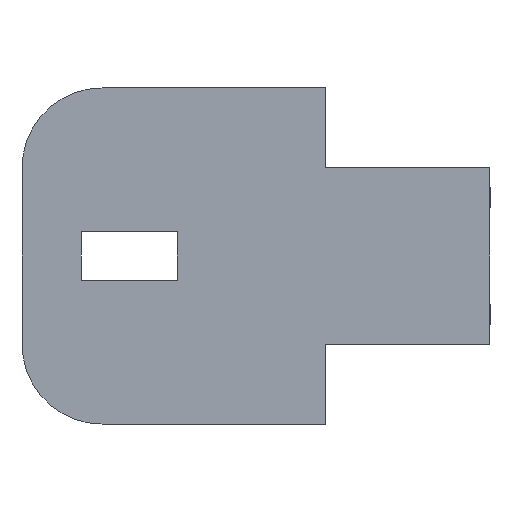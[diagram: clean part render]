
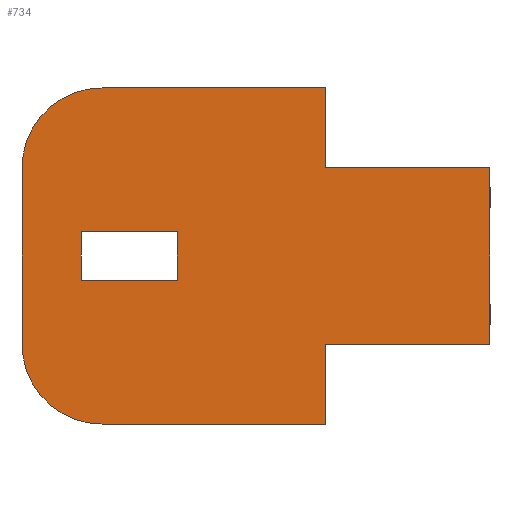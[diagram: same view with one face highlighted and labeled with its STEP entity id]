
A CAD part, left-side view. The second image highlights one B-rep face of the part: STEP entity #734.
In plain terms, the highlighted planar face has unit normal (-1, 0, 0).
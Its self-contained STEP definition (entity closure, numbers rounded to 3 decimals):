
#229=CARTESIAN_POINT('',(-2.155,20.139,4.));
#230=VERTEX_POINT('',#229);
#237=CARTESIAN_POINT('',(-2.155,14.139,4.));
#238=VERTEX_POINT('',#237);
#239=CARTESIAN_POINT('',(-2.155,14.139,4.));
#240=DIRECTION('',(0.0,1.0,0.0));
#241=VECTOR('',#240,6.);
#242=LINE('',#239,#241);
#243=EDGE_CURVE('',#238,#230,#242,.T.);
#260=CARTESIAN_POINT('',(-2.155,20.139,7.));
#261=VERTEX_POINT('',#260);
#268=CARTESIAN_POINT('',(-2.155,20.139,4.));
#269=DIRECTION('',(0.0,0.0,1.0));
#270=VECTOR('',#269,3.);
#271=LINE('',#268,#270);
#272=EDGE_CURVE('',#230,#261,#271,.T.);
#294=CARTESIAN_POINT('',(-2.155,23.839,0.0));
#295=VERTEX_POINT('',#294);
#302=CARTESIAN_POINT('',(-2.155,23.839,11.));
#303=VERTEX_POINT('',#302);
#304=CARTESIAN_POINT('',(-2.155,23.839,0.0));
#305=DIRECTION('',(0.0,0.0,1.0));
#306=VECTOR('',#305,11.);
#307=LINE('',#304,#306);
#308=EDGE_CURVE('',#295,#303,#307,.T.);
#464=CARTESIAN_POINT('',(-2.155,-5.396,11.0));
#465=VERTEX_POINT('',#464);
#472=CARTESIAN_POINT('',(-2.155,-5.396,0.0));
#473=VERTEX_POINT('',#472);
#474=CARTESIAN_POINT('',(-2.155,-5.396,0.0));
#475=DIRECTION('',(0.0,0.0,1.0));
#476=VECTOR('',#475,11.0);
#477=LINE('',#474,#476);
#478=EDGE_CURVE('',#473,#465,#477,.T.);
#574=CARTESIAN_POINT('',(-2.155,14.139,7.));
#575=VERTEX_POINT('',#574);
#582=CARTESIAN_POINT('',(-2.155,20.139,7.));
#583=DIRECTION('',(0.0,-1.0,0.0));
#584=VECTOR('',#583,6.0);
#585=LINE('',#582,#584);
#586=EDGE_CURVE('',#261,#575,#585,.T.);
#599=CARTESIAN_POINT('',(-2.155,14.139,7.));
#600=DIRECTION('',(0.0,0.0,-1.0));
#601=VECTOR('',#600,3.0);
#602=LINE('',#599,#601);
#603=EDGE_CURVE('',#575,#238,#602,.T.);
#614=CARTESIAN_POINT('',(-2.155,18.839,16.0));
#615=VERTEX_POINT('',#614);
#616=CARTESIAN_POINT('',(-2.155,18.839,11.));
#617=DIRECTION('',(1.0,0.,0.));
#618=DIRECTION('',(0.,0.707,0.707));
#619=AXIS2_PLACEMENT_3D('',#616,#617,#618);
#620=CIRCLE('',#619,5.);
#621=EDGE_CURVE('',#303,#615,#620,.T.);
#648=CARTESIAN_POINT('',(-2.155,4.867,16.0));
#649=VERTEX_POINT('',#648);
#650=CARTESIAN_POINT('',(-2.155,18.839,16.0));
#651=DIRECTION('',(0.0,-1.0,0.0));
#652=VECTOR('',#651,13.972);
#653=LINE('',#650,#652);
#654=EDGE_CURVE('',#615,#649,#653,.T.);
#672=CARTESIAN_POINT('',(-2.155,23.839,0.0));
#673=DIRECTION('',(-1.0,0.0,0.0));
#674=DIRECTION('',(0.0,-1.0,0.0));
#675=AXIS2_PLACEMENT_3D('',#672,#673,#674);
#676=PLANE('',#675);
#677=ORIENTED_EDGE('',*,*,#478,.T.);
#678=CARTESIAN_POINT('',(-2.155,4.867,11.0));
#679=VERTEX_POINT('',#678);
#680=CARTESIAN_POINT('',(-2.155,4.867,11.0));
#681=DIRECTION('',(0.0,-1.0,0.0));
#682=VECTOR('',#681,10.263);
#683=LINE('',#680,#682);
#684=EDGE_CURVE('',#679,#465,#683,.T.);
#685=ORIENTED_EDGE('',*,*,#684,.F.);
#686=CARTESIAN_POINT('',(-2.155,4.867,11.0));
#687=DIRECTION('',(0.0,0.0,1.0));
#688=VECTOR('',#687,5.0);
#689=LINE('',#686,#688);
#690=EDGE_CURVE('',#679,#649,#689,.T.);
#691=ORIENTED_EDGE('',*,*,#690,.T.);
#692=ORIENTED_EDGE('',*,*,#654,.F.);
#693=ORIENTED_EDGE('',*,*,#621,.F.);
#694=ORIENTED_EDGE('',*,*,#308,.F.);
#695=CARTESIAN_POINT('',(-2.155,18.839,-5.0));
#696=VERTEX_POINT('',#695);
#697=CARTESIAN_POINT('',(-2.155,18.839,0.0));
#698=DIRECTION('',(1.0,0.,0.));
#699=DIRECTION('',(0.,0.707,-0.707));
#700=AXIS2_PLACEMENT_3D('',#697,#698,#699);
#701=CIRCLE('',#700,5.);
#702=EDGE_CURVE('',#696,#295,#701,.T.);
#703=ORIENTED_EDGE('',*,*,#702,.F.);
#704=CARTESIAN_POINT('',(-2.155,4.904,-5.0));
#705=VERTEX_POINT('',#704);
#706=CARTESIAN_POINT('',(-2.155,4.904,-5.0));
#707=DIRECTION('',(0.0,1.0,0.0));
#708=VECTOR('',#707,13.935);
#709=LINE('',#706,#708);
#710=EDGE_CURVE('',#705,#696,#709,.T.);
#711=ORIENTED_EDGE('',*,*,#710,.F.);
#712=CARTESIAN_POINT('',(-2.155,4.904,0.0));
#713=VERTEX_POINT('',#712);
#714=CARTESIAN_POINT('',(-2.155,4.904,0.0));
#715=DIRECTION('',(0.0,0.0,-1.0));
#716=VECTOR('',#715,5.0);
#717=LINE('',#714,#716);
#718=EDGE_CURVE('',#713,#705,#717,.T.);
#719=ORIENTED_EDGE('',*,*,#718,.F.);
#720=CARTESIAN_POINT('',(-2.155,4.904,0.0));
#721=DIRECTION('',(0.0,-1.0,0.0));
#722=VECTOR('',#721,10.3);
#723=LINE('',#720,#722);
#724=EDGE_CURVE('',#713,#473,#723,.T.);
#725=ORIENTED_EDGE('',*,*,#724,.T.);
#726=EDGE_LOOP('',(#677,#685,#691,#692,#693,#694,#703,#711,#719,#725));
#727=FACE_OUTER_BOUND('',#726,.T.);
#728=ORIENTED_EDGE('',*,*,#586,.T.);
#729=ORIENTED_EDGE('',*,*,#603,.T.);
#730=ORIENTED_EDGE('',*,*,#243,.T.);
#731=ORIENTED_EDGE('',*,*,#272,.T.);
#732=EDGE_LOOP('',(#728,#729,#730,#731));
#733=FACE_BOUND('',#732,.T.);
#734=ADVANCED_FACE('',(#727,#733),#676,.T.);
